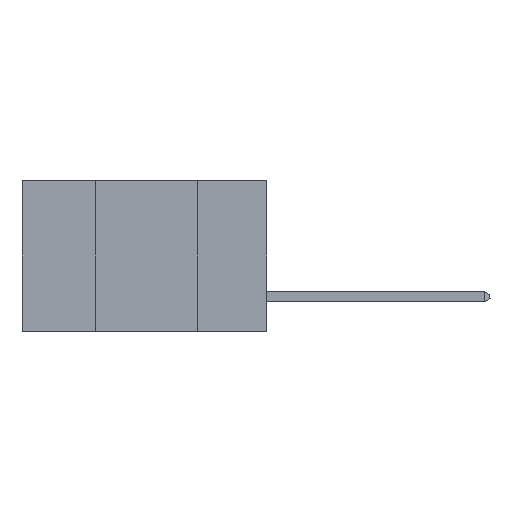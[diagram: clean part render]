
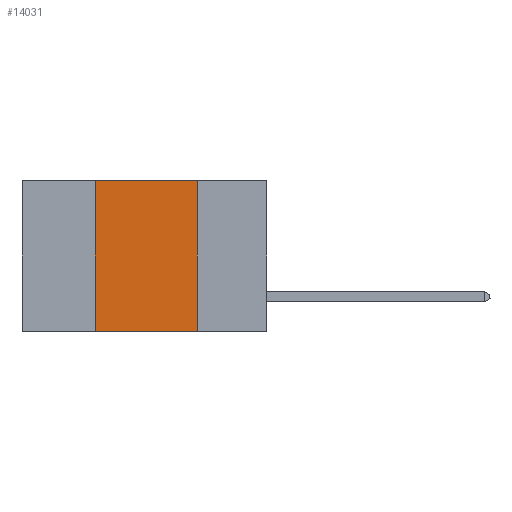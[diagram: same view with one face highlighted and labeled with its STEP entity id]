
A CAD part, left-side view. The second image highlights one B-rep face of the part: STEP entity #14031.
In plain terms, the highlighted planar face has unit normal (-1, 0, 0).
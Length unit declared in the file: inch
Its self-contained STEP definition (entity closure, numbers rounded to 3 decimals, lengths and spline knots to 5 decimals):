
#1087 = ORIENTED_EDGE ( 'NONE', *, *, #7022, .T. ) ;
#1125 = DIRECTION ( 'NONE',  ( 0., -1., 0. ) ) ;
#1298 = LINE ( 'NONE', #7953, #3493 ) ;
#1456 = CARTESIAN_POINT ( 'NONE',  ( 0., 0.42, 0. ) ) ;
#1782 = CARTESIAN_POINT ( 'NONE',  ( 0., 0.17, 0. ) ) ;
#1858 = LINE ( 'NONE', #2524, #5848 ) ;
#2352 = EDGE_LOOP ( 'NONE', ( #10603, #3988, #7107, #1087 ) ) ;
#2524 = CARTESIAN_POINT ( 'NONE',  ( 0., 0.17, 0. ) ) ;
#3493 = VECTOR ( 'NONE', #14902, 39.37008 ) ;
#3627 = EDGE_CURVE ( 'NONE', #11114, #6371, #1858, .T. ) ;
#3988 = ORIENTED_EDGE ( 'NONE', *, *, #4392, .F. ) ;
#4348 = VECTOR ( 'NONE', #12243, 39.37008 ) ;
#4392 = EDGE_CURVE ( 'NONE', #7247, #11114, #12331, .T. ) ;
#5243 = FACE_OUTER_BOUND ( 'NONE', #2352, .T. ) ;
#5848 = VECTOR ( 'NONE', #14108, 39.37008 ) ;
#6371 = VERTEX_POINT ( 'NONE', #14142 ) ;
#7022 = EDGE_CURVE ( 'NONE', #13018, #6371, #14913, .T. ) ;
#7107 = ORIENTED_EDGE ( 'NONE', *, *, #11278, .F. ) ;
#7247 = VERTEX_POINT ( 'NONE', #1456 ) ;
#7953 = CARTESIAN_POINT ( 'NONE',  ( 0., 0.42, 0. ) ) ;
#8427 = PLANE ( 'NONE',  #13985 ) ;
#8438 = CARTESIAN_POINT ( 'NONE',  ( 0., 0.42, -0.37 ) ) ;
#8483 = VECTOR ( 'NONE', #1125, 39.37008 ) ;
#9845 = CARTESIAN_POINT ( 'NONE',  ( 0., 0.6, -0.37 ) ) ;
#10603 = ORIENTED_EDGE ( 'NONE', *, *, #3627, .F. ) ;
#11114 = VERTEX_POINT ( 'NONE', #1782 ) ;
#11278 = EDGE_CURVE ( 'NONE', #13018, #7247, #1298, .T. ) ;
#12195 = DIRECTION ( 'NONE',  ( 1., 0., 0. ) ) ;
#12243 = DIRECTION ( 'NONE',  ( 0., -1., 0. ) ) ;
#12331 = LINE ( 'NONE', #12997, #8483 ) ;
#12997 = CARTESIAN_POINT ( 'NONE',  ( 0., 0.6, 0. ) ) ;
#13018 = VERTEX_POINT ( 'NONE', #8438 ) ;
#13985 = AXIS2_PLACEMENT_3D ( 'NONE', #14245, #12195, #14352 ) ;
#14031 = ADVANCED_FACE ( 'NONE', ( #5243 ), #8427, .F. ) ;
#14108 = DIRECTION ( 'NONE',  ( 0., 0., -1. ) ) ;
#14142 = CARTESIAN_POINT ( 'NONE',  ( 0., 0.17, -0.37 ) ) ;
#14245 = CARTESIAN_POINT ( 'NONE',  ( 0., 0.6, 0. ) ) ;
#14352 = DIRECTION ( 'NONE',  ( 0., 0., -1. ) ) ;
#14902 = DIRECTION ( 'NONE',  ( 0., 0., 1. ) ) ;
#14913 = LINE ( 'NONE', #9845, #4348 ) ;
